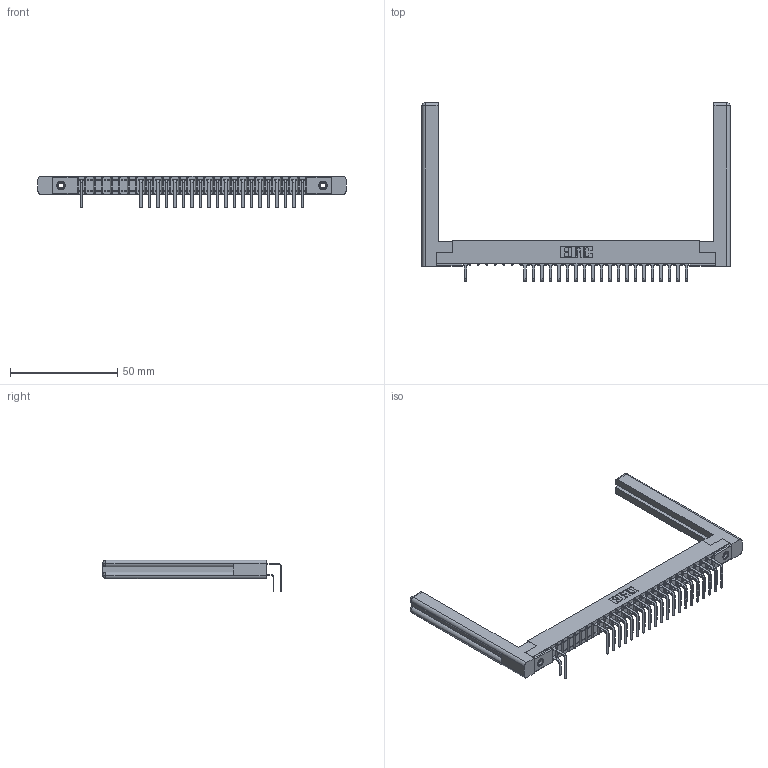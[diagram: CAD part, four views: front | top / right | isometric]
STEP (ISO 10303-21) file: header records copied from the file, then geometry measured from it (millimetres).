
FILE_DESCRIPTION (( 'STEP AP203' ), '1' );
FILE_NAME ('307-027-558-158.STEP', '2018-08-04T15:14:33', ( '' ), ( '' ), 'SwSTEP 2.0', 'SolidWorks 2016', '' );
FILE_SCHEMA (( 'CONFIG_CONTROL_DESIGN' ));
Length unit declared in the file: inch
Products named in the file (6): 307 Part_.156 Dia Mounting Holes; 307-290-001_558 559 - 1 (Single); 307-290-001_558 - 2 (Single); 307-220-058; 345-250-001_345-250-001-102; 307-027-558-158
Assembly tree (46 placements, depth 2):
  307-027-558-158
    307 Part_.156 Dia Mounting Holes
    307-290-001_558 559 - 1 (Single)  x20
    307-290-001_558 - 2 (Single)  x21
    307-220-058  x2
    345-250-001_345-250-001-102  x2
Bounding box: 143.61 x 83.27 x 14.81 mm (x, y, z)
Volume: 17094.9 mm3; surface area: 22006.7 mm2
Topology: 46 solids, 46 shells, 2468 faces, 6915 edges, 4466 vertices
Faces by surface type: plane 1585, cylinder 803, sphere 56, torus 12, cone 12
Entity records: 29524 total; most frequent: CARTESIAN_POINT 4911, ORIENTED_EDGE 4820, DIRECTION 4760, EDGE_CURVE 2410, VECTOR 1838, LINE 1838, VERTEX_POINT 1558, AXIS2_PLACEMENT_3D 1461
